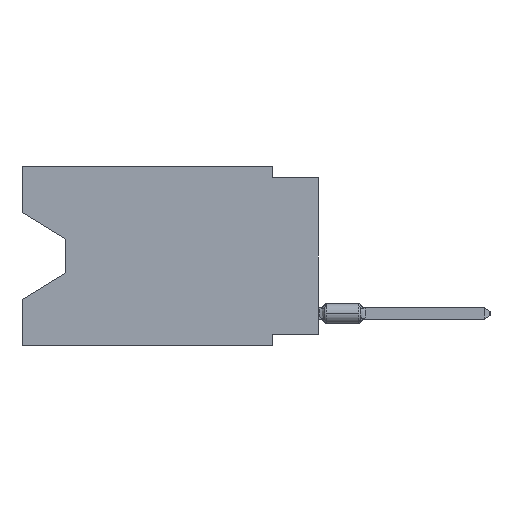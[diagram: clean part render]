
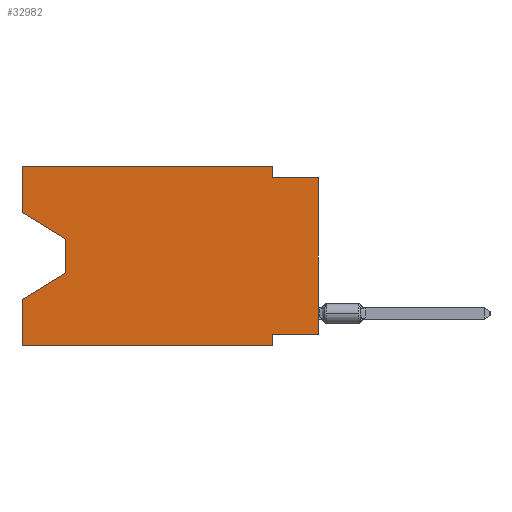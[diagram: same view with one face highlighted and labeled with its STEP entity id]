
A CAD part, left-side view. The second image highlights one B-rep face of the part: STEP entity #32982.
In plain terms, the highlighted planar face has unit normal (-1, 0, 0).
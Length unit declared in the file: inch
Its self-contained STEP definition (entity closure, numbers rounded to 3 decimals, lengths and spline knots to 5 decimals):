
#167 = LINE ( 'NONE', #12010, #23182 ) ;
#307 = EDGE_CURVE ( 'NONE', #19945, #35387, #3630, .T. ) ;
#762 = LINE ( 'NONE', #3320, #34948 ) ;
#1460 = VECTOR ( 'NONE', #4431, 39.37008 ) ;
#1674 = LINE ( 'NONE', #4422, #9755 ) ;
#2515 = VERTEX_POINT ( 'NONE', #24612 ) ;
#3320 = CARTESIAN_POINT ( 'NONE',  ( 0., 0.645, -0.39 ) ) ;
#3476 = CARTESIAN_POINT ( 'NONE',  ( 0., 0.1, -0.39 ) ) ;
#3535 = VERTEX_POINT ( 'NONE', #15031 ) ;
#3630 = LINE ( 'NONE', #9636, #13299 ) ;
#4422 = CARTESIAN_POINT ( 'NONE',  ( 0., 0.645, 0. ) ) ;
#4431 = DIRECTION ( 'NONE',  ( 0., 0., 1. ) ) ;
#4446 = ORIENTED_EDGE ( 'NONE', *, *, #30439, .F. ) ;
#4793 = LINE ( 'NONE', #35805, #22399 ) ;
#5002 = CARTESIAN_POINT ( 'NONE',  ( 0., 0., -0.025 ) ) ;
#5262 = ORIENTED_EDGE ( 'NONE', *, *, #35661, .F. ) ;
#5568 = CARTESIAN_POINT ( 'NONE',  ( 0., 0.55, -0.232 ) ) ;
#5880 = AXIS2_PLACEMENT_3D ( 'NONE', #26182, #31495, #6488 ) ;
#6488 = DIRECTION ( 'NONE',  ( 0., 0., -1. ) ) ;
#6610 = DIRECTION ( 'NONE',  ( 0., -1., 0. ) ) ;
#6870 = ORIENTED_EDGE ( 'NONE', *, *, #24188, .F. ) ;
#6984 = CARTESIAN_POINT ( 'NONE',  ( 0., 0., 0. ) ) ;
#7738 = ORIENTED_EDGE ( 'NONE', *, *, #34852, .T. ) ;
#7944 = ORIENTED_EDGE ( 'NONE', *, *, #30852, .T. ) ;
#8132 = VERTEX_POINT ( 'NONE', #21829 ) ;
#8623 = VERTEX_POINT ( 'NONE', #5568 ) ;
#8748 = VECTOR ( 'NONE', #27441, 39.37008 ) ;
#9007 = CARTESIAN_POINT ( 'NONE',  ( 0., 0.645, -0.10025 ) ) ;
#9086 = CARTESIAN_POINT ( 'NONE',  ( 0., 0.55, -0.158 ) ) ;
#9636 = CARTESIAN_POINT ( 'NONE',  ( 0., 0., -0.365 ) ) ;
#9755 = VECTOR ( 'NONE', #29061, 39.37008 ) ;
#10498 = EDGE_CURVE ( 'NONE', #3535, #8132, #1674, .T. ) ;
#10831 = VECTOR ( 'NONE', #25722, 39.37008 ) ;
#11339 = VERTEX_POINT ( 'NONE', #5002 ) ;
#11481 = CARTESIAN_POINT ( 'NONE',  ( 0., 0.1, 0. ) ) ;
#12010 = CARTESIAN_POINT ( 'NONE',  ( 0., 0.645, 0. ) ) ;
#12186 = CARTESIAN_POINT ( 'NONE',  ( 0., 0.1, 0. ) ) ;
#12474 = EDGE_CURVE ( 'NONE', #8623, #8132, #26316, .T. ) ;
#13153 = LINE ( 'NONE', #6984, #1460 ) ;
#13299 = VECTOR ( 'NONE', #20743, 39.37008 ) ;
#13706 = DIRECTION ( 'NONE',  ( 0., 0., 1. ) ) ;
#13911 = VECTOR ( 'NONE', #24103, 39.37008 ) ;
#14044 = LINE ( 'NONE', #11481, #10831 ) ;
#14508 = LINE ( 'NONE', #31496, #35266 ) ;
#14734 = CARTESIAN_POINT ( 'NONE',  ( 0., 0.645, -0.10025 ) ) ;
#15031 = CARTESIAN_POINT ( 'NONE',  ( 0., 0.645, -0.39 ) ) ;
#15463 = VERTEX_POINT ( 'NONE', #32556 ) ;
#16971 = VERTEX_POINT ( 'NONE', #12186 ) ;
#17940 = CARTESIAN_POINT ( 'NONE',  ( 0., 0., -0.025 ) ) ;
#18561 = VECTOR ( 'NONE', #19639, 39.37008 ) ;
#19639 = DIRECTION ( 'NONE',  ( 0., -1., 0. ) ) ;
#19856 = EDGE_CURVE ( 'NONE', #31489, #8623, #14508, .T. ) ;
#19945 = VERTEX_POINT ( 'NONE', #24321 ) ;
#20156 = FACE_OUTER_BOUND ( 'NONE', #26064, .T. ) ;
#20743 = DIRECTION ( 'NONE',  ( 0., 1., 0. ) ) ;
#20772 = EDGE_CURVE ( 'NONE', #22694, #31489, #34108, .T. ) ;
#21455 = ORIENTED_EDGE ( 'NONE', *, *, #32133, .F. ) ;
#21829 = CARTESIAN_POINT ( 'NONE',  ( 0., 0.645, -0.28975 ) ) ;
#22399 = VECTOR ( 'NONE', #13706, 39.37008 ) ;
#22694 = VERTEX_POINT ( 'NONE', #9007 ) ;
#22777 = DIRECTION ( 'NONE',  ( 0., -1., 0. ) ) ;
#22790 = LINE ( 'NONE', #3476, #8748 ) ;
#22842 = ORIENTED_EDGE ( 'NONE', *, *, #19856, .T. ) ;
#22885 = PLANE ( 'NONE',  #5880 ) ;
#23182 = VECTOR ( 'NONE', #22777, 39.37008 ) ;
#24103 = DIRECTION ( 'NONE',  ( 0., 0.855, -0.519 ) ) ;
#24188 = EDGE_CURVE ( 'NONE', #22694, #15463, #4793, .T. ) ;
#24321 = CARTESIAN_POINT ( 'NONE',  ( 0., 0., -0.365 ) ) ;
#24612 = CARTESIAN_POINT ( 'NONE',  ( 0., 0.1, -0.025 ) ) ;
#25722 = DIRECTION ( 'NONE',  ( 0., 0., -1. ) ) ;
#26064 = EDGE_LOOP ( 'NONE', ( #34453, #22842, #29907, #26618, #7944, #21455, #32260, #7738, #4446, #5262, #35808, #6870 ) ) ;
#26182 = CARTESIAN_POINT ( 'NONE',  ( 0., 0.645, 0. ) ) ;
#26316 = LINE ( 'NONE', #26686, #13911 ) ;
#26618 = ORIENTED_EDGE ( 'NONE', *, *, #10498, .F. ) ;
#26686 = CARTESIAN_POINT ( 'NONE',  ( 0., 0.55, -0.232 ) ) ;
#27039 = CARTESIAN_POINT ( 'NONE',  ( 0., 0.1, -0.39 ) ) ;
#27441 = DIRECTION ( 'NONE',  ( 0., 0., -1. ) ) ;
#28749 = VECTOR ( 'NONE', #31721, 39.37008 ) ;
#28873 = CARTESIAN_POINT ( 'NONE',  ( 0., 0.1, -0.365 ) ) ;
#29061 = DIRECTION ( 'NONE',  ( 0., 0., 1. ) ) ;
#29092 = LINE ( 'NONE', #17940, #18561 ) ;
#29907 = ORIENTED_EDGE ( 'NONE', *, *, #12474, .T. ) ;
#29964 = EDGE_CURVE ( 'NONE', #15463, #16971, #167, .T. ) ;
#30439 = EDGE_CURVE ( 'NONE', #2515, #11339, #29092, .T. ) ;
#30852 = EDGE_CURVE ( 'NONE', #3535, #34823, #762, .T. ) ;
#31489 = VERTEX_POINT ( 'NONE', #9086 ) ;
#31495 = DIRECTION ( 'NONE',  ( 1., 0., 0. ) ) ;
#31496 = CARTESIAN_POINT ( 'NONE',  ( 0., 0.55, -0.158 ) ) ;
#31721 = DIRECTION ( 'NONE',  ( 0., -0.855, -0.519 ) ) ;
#32133 = EDGE_CURVE ( 'NONE', #35387, #34823, #22790, .T. ) ;
#32260 = ORIENTED_EDGE ( 'NONE', *, *, #307, .F. ) ;
#32556 = CARTESIAN_POINT ( 'NONE',  ( 0., 0.645, 0. ) ) ;
#32982 = ADVANCED_FACE ( 'NONE', ( #20156 ), #22885, .F. ) ;
#33876 = DIRECTION ( 'NONE',  ( 0., 0., -1. ) ) ;
#34108 = LINE ( 'NONE', #14734, #28749 ) ;
#34453 = ORIENTED_EDGE ( 'NONE', *, *, #20772, .T. ) ;
#34823 = VERTEX_POINT ( 'NONE', #27039 ) ;
#34852 = EDGE_CURVE ( 'NONE', #19945, #11339, #13153, .T. ) ;
#34948 = VECTOR ( 'NONE', #6610, 39.37008 ) ;
#35266 = VECTOR ( 'NONE', #33876, 39.37008 ) ;
#35387 = VERTEX_POINT ( 'NONE', #28873 ) ;
#35661 = EDGE_CURVE ( 'NONE', #16971, #2515, #14044, .T. ) ;
#35805 = CARTESIAN_POINT ( 'NONE',  ( 0., 0.645, 0. ) ) ;
#35808 = ORIENTED_EDGE ( 'NONE', *, *, #29964, .F. ) ;
